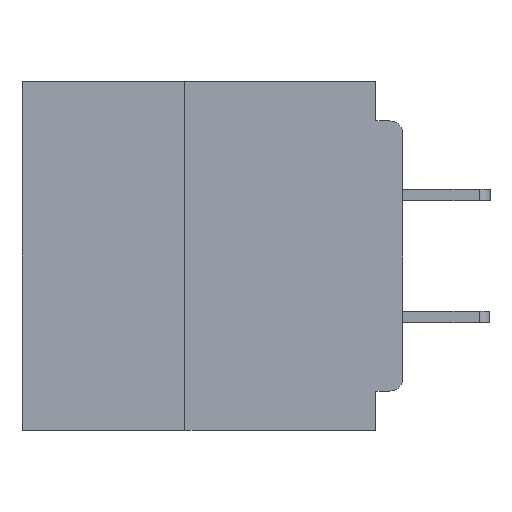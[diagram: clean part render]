
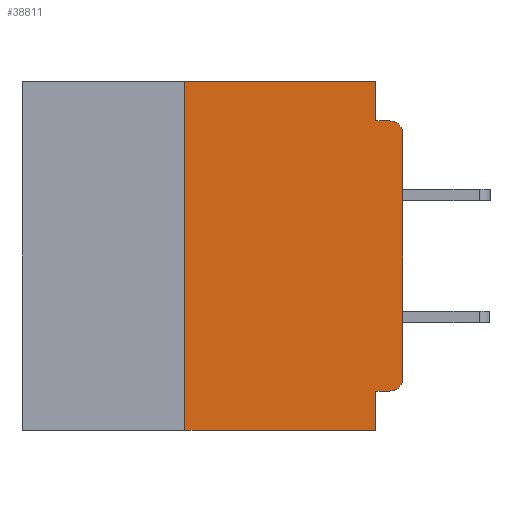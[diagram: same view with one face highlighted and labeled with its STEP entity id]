
A CAD part, left-side view. The second image highlights one B-rep face of the part: STEP entity #38811.
In plain terms, the highlighted planar face has unit normal (-1, 0, 0).
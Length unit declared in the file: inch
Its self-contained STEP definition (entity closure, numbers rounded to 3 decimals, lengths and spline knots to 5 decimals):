
#213 = DIRECTION ( 'NONE',  ( 0., 0., -1. ) ) ;
#534 = CIRCLE ( 'NONE', #7939, 0.015 ) ;
#889 = ORIENTED_EDGE ( 'NONE', *, *, #2656, .T. ) ;
#1193 = DIRECTION ( 'NONE',  ( 0., -1., 0. ) ) ;
#2656 = EDGE_CURVE ( 'NONE', #27464, #7502, #534, .T. ) ;
#3778 = VERTEX_POINT ( 'NONE', #31465 ) ;
#4113 = VERTEX_POINT ( 'NONE', #37421 ) ;
#4916 = ORIENTED_EDGE ( 'NONE', *, *, #16954, .T. ) ;
#6324 = VERTEX_POINT ( 'NONE', #27384 ) ;
#6338 = ORIENTED_EDGE ( 'NONE', *, *, #33591, .F. ) ;
#6454 = EDGE_CURVE ( 'NONE', #14465, #27464, #8226, .T. ) ;
#6988 = ORIENTED_EDGE ( 'NONE', *, *, #6454, .T. ) ;
#7156 = VECTOR ( 'NONE', #34566, 39.37008 ) ;
#7374 = CARTESIAN_POINT ( 'NONE',  ( 0., 0., -0.045 ) ) ;
#7502 = VERTEX_POINT ( 'NONE', #33032 ) ;
#7939 = AXIS2_PLACEMENT_3D ( 'NONE', #36400, #36363, #36347 ) ;
#8195 = DIRECTION ( 'NONE',  ( 1., 0., 0. ) ) ;
#8226 = LINE ( 'NONE', #17998, #7156 ) ;
#8624 = LINE ( 'NONE', #24593, #16553 ) ;
#9219 = LINE ( 'NONE', #7374, #17147 ) ;
#10817 = CARTESIAN_POINT ( 'NONE',  ( 0., 0., -0.355 ) ) ;
#10961 = VERTEX_POINT ( 'NONE', #12432 ) ;
#12048 = ORIENTED_EDGE ( 'NONE', *, *, #19909, .F. ) ;
#12428 = AXIS2_PLACEMENT_3D ( 'NONE', #28356, #8195, #31663 ) ;
#12432 = CARTESIAN_POINT ( 'NONE',  ( 0., 0.25, 0. ) ) ;
#13271 = CARTESIAN_POINT ( 'NONE',  ( 0., 0.031, 0. ) ) ;
#14433 = CARTESIAN_POINT ( 'NONE',  ( 0., 0.015, -0.355 ) ) ;
#14465 = VERTEX_POINT ( 'NONE', #33342 ) ;
#15436 = VECTOR ( 'NONE', #42666, 39.37008 ) ;
#15589 = CARTESIAN_POINT ( 'NONE',  ( 0., 0.031, -0.4 ) ) ;
#16195 = CARTESIAN_POINT ( 'NONE',  ( 0., 0.031, 0. ) ) ;
#16196 = VECTOR ( 'NONE', #1193, 39.37008 ) ;
#16200 = CARTESIAN_POINT ( 'NONE',  ( 0., 0.437, -0.4 ) ) ;
#16262 = VERTEX_POINT ( 'NONE', #29623 ) ;
#16553 = VECTOR ( 'NONE', #17834, 39.37008 ) ;
#16954 = EDGE_CURVE ( 'NONE', #4113, #6324, #36598, .T. ) ;
#17147 = VECTOR ( 'NONE', #34164, 39.37008 ) ;
#17267 = LINE ( 'NONE', #37920, #16196 ) ;
#17348 = CARTESIAN_POINT ( 'NONE',  ( 0., 0., -0.06 ) ) ;
#17632 = DIRECTION ( 'NONE',  ( 0., 1., 0. ) ) ;
#17834 = DIRECTION ( 'NONE',  ( 0., 0., 1. ) ) ;
#17998 = CARTESIAN_POINT ( 'NONE',  ( 0., 0., 0. ) ) ;
#18811 = VECTOR ( 'NONE', #17632, 39.37008 ) ;
#19374 = VERTEX_POINT ( 'NONE', #13271 ) ;
#19909 = EDGE_CURVE ( 'NONE', #19374, #3778, #41861, .T. ) ;
#20516 = DIRECTION ( 'NONE',  ( -1., 0., 0. ) ) ;
#20903 = EDGE_LOOP ( 'NONE', ( #6988, #889, #42832, #12048, #6338, #42933, #4916, #40037, #31372, #22378 ) ) ;
#21664 = PLANE ( 'NONE',  #12428 ) ;
#22378 = ORIENTED_EDGE ( 'NONE', *, *, #32776, .T. ) ;
#22858 = EDGE_CURVE ( 'NONE', #16262, #6324, #43128, .T. ) ;
#23230 = EDGE_CURVE ( 'NONE', #41777, #16262, #36461, .T. ) ;
#23628 = VECTOR ( 'NONE', #25720, 39.37008 ) ;
#24593 = CARTESIAN_POINT ( 'NONE',  ( 0., 0.25, -0.4 ) ) ;
#25720 = DIRECTION ( 'NONE',  ( 0., 0., -1. ) ) ;
#26354 = DIRECTION ( 'NONE',  ( 0., -1., 0. ) ) ;
#26834 = VECTOR ( 'NONE', #26354, 39.37008 ) ;
#27384 = CARTESIAN_POINT ( 'NONE',  ( 0., 0.031, -0.4 ) ) ;
#27464 = VERTEX_POINT ( 'NONE', #17348 ) ;
#28356 = CARTESIAN_POINT ( 'NONE',  ( 0., 0.437, 0. ) ) ;
#29623 = CARTESIAN_POINT ( 'NONE',  ( 0., 0.031, -0.355 ) ) ;
#30004 = AXIS2_PLACEMENT_3D ( 'NONE', #40260, #20516, #213 ) ;
#31372 = ORIENTED_EDGE ( 'NONE', *, *, #23230, .F. ) ;
#31465 = CARTESIAN_POINT ( 'NONE',  ( 0., 0.031, -0.045 ) ) ;
#31663 = DIRECTION ( 'NONE',  ( 0., 0., -1. ) ) ;
#32776 = EDGE_CURVE ( 'NONE', #41777, #14465, #41673, .T. ) ;
#33032 = CARTESIAN_POINT ( 'NONE',  ( 0., 0.015, -0.045 ) ) ;
#33342 = CARTESIAN_POINT ( 'NONE',  ( 0., 0., -0.34 ) ) ;
#33591 = EDGE_CURVE ( 'NONE', #10961, #19374, #17267, .T. ) ;
#34164 = DIRECTION ( 'NONE',  ( 0., -1., 0. ) ) ;
#34566 = DIRECTION ( 'NONE',  ( 0., 0., 1. ) ) ;
#34860 = EDGE_CURVE ( 'NONE', #3778, #7502, #9219, .T. ) ;
#35556 = EDGE_CURVE ( 'NONE', #4113, #10961, #8624, .T. ) ;
#36161 = FACE_OUTER_BOUND ( 'NONE', #20903, .T. ) ;
#36347 = DIRECTION ( 'NONE',  ( 0., 0., -1. ) ) ;
#36363 = DIRECTION ( 'NONE',  ( -1., 0., 0. ) ) ;
#36400 = CARTESIAN_POINT ( 'NONE',  ( 0., 0.015, -0.06 ) ) ;
#36461 = LINE ( 'NONE', #10817, #18811 ) ;
#36598 = LINE ( 'NONE', #16200, #26834 ) ;
#37421 = CARTESIAN_POINT ( 'NONE',  ( 0., 0.25, -0.4 ) ) ;
#37920 = CARTESIAN_POINT ( 'NONE',  ( 0., 0.437, 0. ) ) ;
#38811 = ADVANCED_FACE ( 'NONE', ( #36161 ), #21664, .F. ) ;
#40037 = ORIENTED_EDGE ( 'NONE', *, *, #22858, .F. ) ;
#40260 = CARTESIAN_POINT ( 'NONE',  ( 0., 0.015, -0.34 ) ) ;
#41673 = CIRCLE ( 'NONE', #30004, 0.015 ) ;
#41777 = VERTEX_POINT ( 'NONE', #14433 ) ;
#41861 = LINE ( 'NONE', #16195, #15436 ) ;
#42666 = DIRECTION ( 'NONE',  ( 0., 0., -1. ) ) ;
#42832 = ORIENTED_EDGE ( 'NONE', *, *, #34860, .F. ) ;
#42933 = ORIENTED_EDGE ( 'NONE', *, *, #35556, .F. ) ;
#43128 = LINE ( 'NONE', #15589, #23628 ) ;
